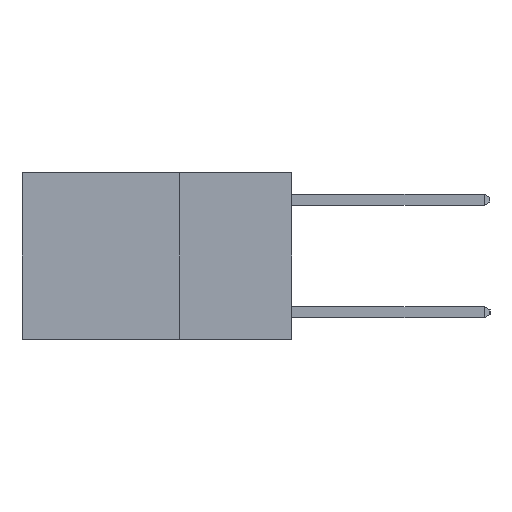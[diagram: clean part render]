
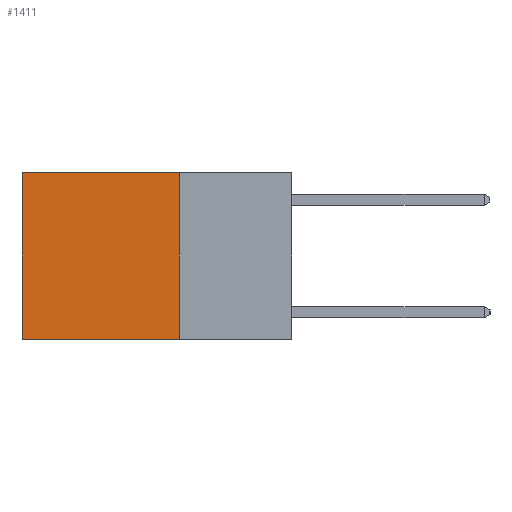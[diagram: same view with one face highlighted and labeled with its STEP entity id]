
A CAD part, left-side view. The second image highlights one B-rep face of the part: STEP entity #1411.
In plain terms, the highlighted planar face has unit normal (-1, 0, 0).
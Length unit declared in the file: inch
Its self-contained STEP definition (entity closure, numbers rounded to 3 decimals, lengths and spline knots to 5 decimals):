
#946 = VERTEX_POINT ( 'NONE', #3892 ) ;
#1029 = DIRECTION ( 'NONE',  ( 0., 1., 0. ) ) ;
#1134 = ORIENTED_EDGE ( 'NONE', *, *, #9898, .F. ) ;
#1166 = LINE ( 'NONE', #3710, #5509 ) ;
#1202 = DIRECTION ( 'NONE',  ( 0., 1., 0. ) ) ;
#1403 = EDGE_CURVE ( 'NONE', #3349, #946, #2894, .T. ) ;
#1411 = ADVANCED_FACE ( 'NONE', ( #9054 ), #10092, .F. ) ;
#1774 = VERTEX_POINT ( 'NONE', #9906 ) ;
#2116 = DIRECTION ( 'NONE',  ( 0., 0., -1. ) ) ;
#2401 = AXIS2_PLACEMENT_3D ( 'NONE', #8332, #3530, #8422 ) ;
#2894 = LINE ( 'NONE', #3617, #7267 ) ;
#3349 = VERTEX_POINT ( 'NONE', #6659 ) ;
#3488 = EDGE_LOOP ( 'NONE', ( #7899, #1134, #8120, #5070 ) ) ;
#3530 = DIRECTION ( 'NONE',  ( 1., 0., 0. ) ) ;
#3570 = EDGE_CURVE ( 'NONE', #3349, #5668, #1166, .T. ) ;
#3617 = CARTESIAN_POINT ( 'NONE',  ( 0.2625, 0.25, 0. ) ) ;
#3710 = CARTESIAN_POINT ( 'NONE',  ( 0.2625, 0.25, 0. ) ) ;
#3734 = LINE ( 'NONE', #7104, #10500 ) ;
#3892 = CARTESIAN_POINT ( 'NONE',  ( 0.2625, 0.25, -0.37 ) ) ;
#4767 = CARTESIAN_POINT ( 'NONE',  ( 0.2625, 0.6, 0. ) ) ;
#5070 = ORIENTED_EDGE ( 'NONE', *, *, #3570, .T. ) ;
#5509 = VECTOR ( 'NONE', #1029, 39.37008 ) ;
#5548 = VECTOR ( 'NONE', #1202, 39.37008 ) ;
#5668 = VERTEX_POINT ( 'NONE', #4767 ) ;
#5810 = LINE ( 'NONE', #8600, #5548 ) ;
#6659 = CARTESIAN_POINT ( 'NONE',  ( 0.2625, 0.25, 0. ) ) ;
#7104 = CARTESIAN_POINT ( 'NONE',  ( 0.2625, 0.6, 0. ) ) ;
#7267 = VECTOR ( 'NONE', #9538, 39.37008 ) ;
#7899 = ORIENTED_EDGE ( 'NONE', *, *, #9273, .T. ) ;
#8120 = ORIENTED_EDGE ( 'NONE', *, *, #1403, .F. ) ;
#8332 = CARTESIAN_POINT ( 'NONE',  ( 0.2625, 0.25, 0. ) ) ;
#8422 = DIRECTION ( 'NONE',  ( 0., 0., -1. ) ) ;
#8600 = CARTESIAN_POINT ( 'NONE',  ( 0.2625, 0.25, -0.37 ) ) ;
#9054 = FACE_OUTER_BOUND ( 'NONE', #3488, .T. ) ;
#9273 = EDGE_CURVE ( 'NONE', #5668, #1774, #3734, .T. ) ;
#9538 = DIRECTION ( 'NONE',  ( 0., 0., -1. ) ) ;
#9898 = EDGE_CURVE ( 'NONE', #946, #1774, #5810, .T. ) ;
#9906 = CARTESIAN_POINT ( 'NONE',  ( 0.2625, 0.6, -0.37 ) ) ;
#10092 = PLANE ( 'NONE',  #2401 ) ;
#10500 = VECTOR ( 'NONE', #2116, 39.37008 ) ;
